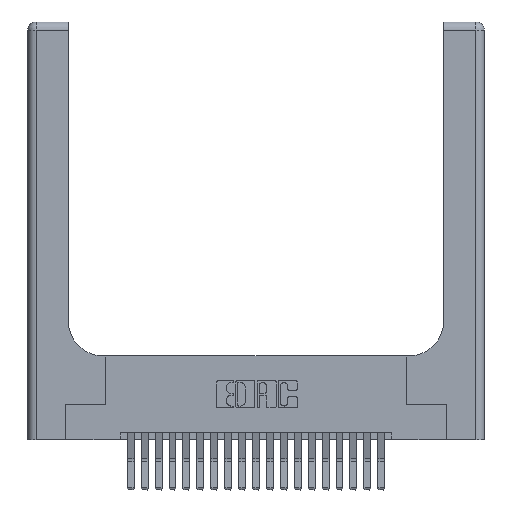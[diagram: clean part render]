
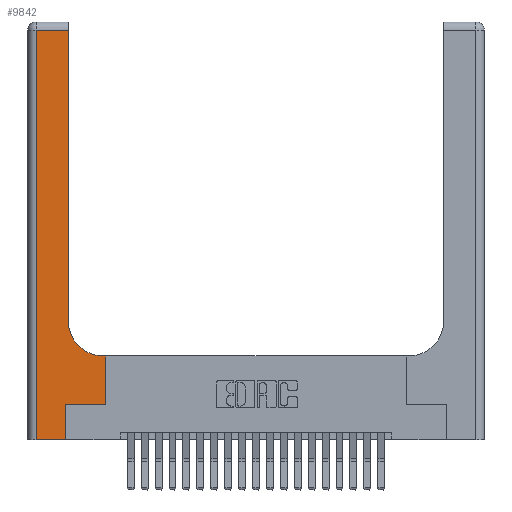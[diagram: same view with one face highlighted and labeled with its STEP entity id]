
A CAD part, top view. The second image highlights one B-rep face of the part: STEP entity #9842.
In plain terms, the highlighted planar face has unit normal (0, 0, 1).
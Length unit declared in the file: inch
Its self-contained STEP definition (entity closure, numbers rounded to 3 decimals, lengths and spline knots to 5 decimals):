
#53 = VECTOR ( 'NONE', #16639, 39.37008 ) ;
#1067 = ORIENTED_EDGE ( 'NONE', *, *, #2316, .T. ) ;
#1154 = ORIENTED_EDGE ( 'NONE', *, *, #15011, .T. ) ;
#1434 = ORIENTED_EDGE ( 'NONE', *, *, #15680, .T. ) ;
#1575 = ORIENTED_EDGE ( 'NONE', *, *, #2482, .T. ) ;
#1633 = CARTESIAN_POINT ( 'NONE',  ( 0.2915, 0.6, 0.37 ) ) ;
#2050 = CARTESIAN_POINT ( 'NONE',  ( 0.5415, 0.6, 0.37 ) ) ;
#2316 = EDGE_CURVE ( 'NONE', #11499, #21631, #12574, .T. ) ;
#2482 = EDGE_CURVE ( 'NONE', #6622, #8612, #22486, .T. ) ;
#3942 = EDGE_CURVE ( 'NONE', #21631, #12793, #5821, .T. ) ;
#4805 = LINE ( 'NONE', #16977, #14029 ) ;
#4995 = CARTESIAN_POINT ( 'NONE',  ( 0.269, 0.25, 0.37 ) ) ;
#5080 = DIRECTION ( 'NONE',  ( 1., 0., 0. ) ) ;
#5223 = FACE_OUTER_BOUND ( 'NONE', #16243, .T. ) ;
#5552 = DIRECTION ( 'NONE',  ( 0., 0., -1. ) ) ;
#5705 = LINE ( 'NONE', #16568, #53 ) ;
#5806 = ORIENTED_EDGE ( 'NONE', *, *, #5961, .T. ) ;
#5821 = LINE ( 'NONE', #11482, #14966 ) ;
#5907 = ORIENTED_EDGE ( 'NONE', *, *, #20732, .T. ) ;
#5961 = EDGE_CURVE ( 'NONE', #10531, #11499, #23184, .T. ) ;
#5983 = VECTOR ( 'NONE', #7147, 39.37008 ) ;
#6602 = LINE ( 'NONE', #19496, #5983 ) ;
#6622 = VERTEX_POINT ( 'NONE', #9229 ) ;
#7147 = DIRECTION ( 'NONE',  ( 0., 1., 0. ) ) ;
#8143 = VERTEX_POINT ( 'NONE', #23278 ) ;
#8612 = VERTEX_POINT ( 'NONE', #21196 ) ;
#9201 = DIRECTION ( 'NONE',  ( 0., 1., 0. ) ) ;
#9229 = CARTESIAN_POINT ( 'NONE',  ( 0.269, 0.25, 0.37 ) ) ;
#9283 = CARTESIAN_POINT ( 'NONE',  ( 0.06, 2.94, 0.37 ) ) ;
#9345 = AXIS2_PLACEMENT_3D ( 'NONE', #14496, #10862, #17971 ) ;
#9842 = ADVANCED_FACE ( 'NONE', ( #5223 ), #16233, .F. ) ;
#9886 = ORIENTED_EDGE ( 'NONE', *, *, #11998, .T. ) ;
#10531 = VERTEX_POINT ( 'NONE', #2050 ) ;
#10581 = CARTESIAN_POINT ( 'NONE',  ( 0.5585, 0.6, 0.37 ) ) ;
#10862 = DIRECTION ( 'NONE',  ( 0., 0., -1. ) ) ;
#11246 = ORIENTED_EDGE ( 'NONE', *, *, #20030, .T. ) ;
#11482 = CARTESIAN_POINT ( 'NONE',  ( 0., 2.94, 0.37 ) ) ;
#11499 = VERTEX_POINT ( 'NONE', #19950 ) ;
#11980 = VECTOR ( 'NONE', #18903, 39.37008 ) ;
#11998 = EDGE_CURVE ( 'NONE', #8143, #6622, #6602, .T. ) ;
#12574 = LINE ( 'NONE', #20622, #11980 ) ;
#12793 = VERTEX_POINT ( 'NONE', #9283 ) ;
#13339 = DIRECTION ( 'NONE',  ( -1., 0., 0. ) ) ;
#13578 = DIRECTION ( 'NONE',  ( 0., -1., 0. ) ) ;
#14029 = VECTOR ( 'NONE', #13578, 39.37008 ) ;
#14055 = CARTESIAN_POINT ( 'NONE',  ( 0.06, 0., 0.37 ) ) ;
#14496 = CARTESIAN_POINT ( 'NONE',  ( 0., 3., 0.37 ) ) ;
#14966 = VECTOR ( 'NONE', #13339, 39.37008 ) ;
#15011 = EDGE_CURVE ( 'NONE', #22139, #10531, #20658, .T. ) ;
#15680 = EDGE_CURVE ( 'NONE', #8612, #22139, #16123, .T. ) ;
#15837 = CARTESIAN_POINT ( 'NONE',  ( 0.2915, 2.94, 0.37 ) ) ;
#16123 = LINE ( 'NONE', #16303, #20144 ) ;
#16233 = PLANE ( 'NONE',  #9345 ) ;
#16243 = EDGE_LOOP ( 'NONE', ( #1067, #19975, #5907, #11246, #9886, #1575, #1434, #1154, #5806 ) ) ;
#16303 = CARTESIAN_POINT ( 'NONE',  ( 0.5585, 0.25, 0.37 ) ) ;
#16429 = CARTESIAN_POINT ( 'NONE',  ( 0.5415, 0.85, 0.37 ) ) ;
#16568 = CARTESIAN_POINT ( 'NONE',  ( 0., 0., 0.37 ) ) ;
#16639 = DIRECTION ( 'NONE',  ( 1., 0., 0. ) ) ;
#16977 = CARTESIAN_POINT ( 'NONE',  ( 0.06, 3., 0.37 ) ) ;
#17971 = DIRECTION ( 'NONE',  ( -1., 0., 0. ) ) ;
#18008 = VECTOR ( 'NONE', #5080, 39.37008 ) ;
#18065 = DIRECTION ( 'NONE',  ( -1., 0., 0. ) ) ;
#18164 = DIRECTION ( 'NONE',  ( 1., 0., 0. ) ) ;
#18521 = VERTEX_POINT ( 'NONE', #14055 ) ;
#18903 = DIRECTION ( 'NONE',  ( 0., 1., 0. ) ) ;
#19496 = CARTESIAN_POINT ( 'NONE',  ( 0.269, 0., 0.37 ) ) ;
#19950 = CARTESIAN_POINT ( 'NONE',  ( 0.2915, 0.85, 0.37 ) ) ;
#19975 = ORIENTED_EDGE ( 'NONE', *, *, #3942, .T. ) ;
#20030 = EDGE_CURVE ( 'NONE', #18521, #8143, #5705, .T. ) ;
#20144 = VECTOR ( 'NONE', #9201, 39.37008 ) ;
#20622 = CARTESIAN_POINT ( 'NONE',  ( 0.2915, 3., 0.37 ) ) ;
#20658 = LINE ( 'NONE', #1633, #22728 ) ;
#20732 = EDGE_CURVE ( 'NONE', #12793, #18521, #4805, .T. ) ;
#21196 = CARTESIAN_POINT ( 'NONE',  ( 0.5585, 0.25, 0.37 ) ) ;
#21631 = VERTEX_POINT ( 'NONE', #15837 ) ;
#22139 = VERTEX_POINT ( 'NONE', #10581 ) ;
#22415 = AXIS2_PLACEMENT_3D ( 'NONE', #16429, #5552, #18164 ) ;
#22486 = LINE ( 'NONE', #4995, #18008 ) ;
#22728 = VECTOR ( 'NONE', #18065, 39.37008 ) ;
#23184 = CIRCLE ( 'NONE', #22415, 0.25 ) ;
#23278 = CARTESIAN_POINT ( 'NONE',  ( 0.269, 0., 0.37 ) ) ;
